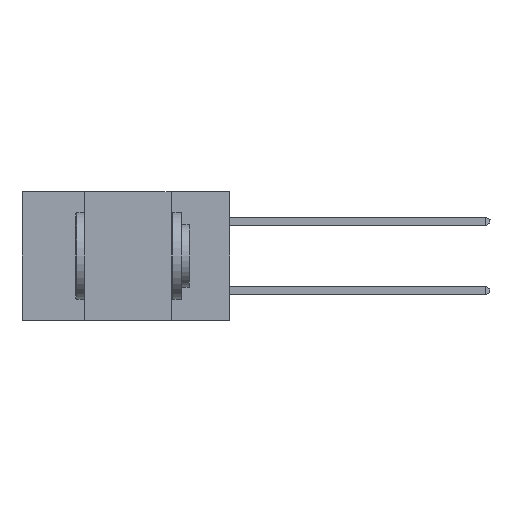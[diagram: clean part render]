
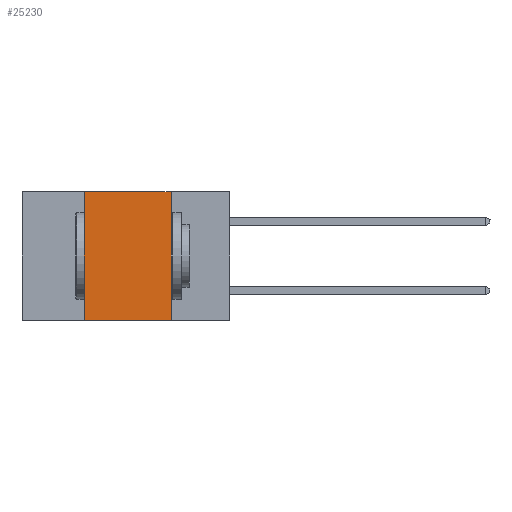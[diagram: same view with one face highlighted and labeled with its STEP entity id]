
A CAD part, left-side view. The second image highlights one B-rep face of the part: STEP entity #25230.
In plain terms, the highlighted planar face has unit normal (-1, 0, 0).
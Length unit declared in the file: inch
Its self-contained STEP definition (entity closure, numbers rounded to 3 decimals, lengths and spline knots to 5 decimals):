
#1591 = CARTESIAN_POINT ( 'NONE',  ( 0., 0.42, 0. ) ) ;
#3230 = VECTOR ( 'NONE', #23755, 39.37008 ) ;
#4613 = EDGE_LOOP ( 'NONE', ( #8569, #6033, #12265, #22360 ) ) ;
#5882 = VECTOR ( 'NONE', #16762, 39.37008 ) ;
#6033 = ORIENTED_EDGE ( 'NONE', *, *, #14256, .F. ) ;
#6796 = CARTESIAN_POINT ( 'NONE',  ( 0., 0.42, 0. ) ) ;
#7136 = VERTEX_POINT ( 'NONE', #1591 ) ;
#8569 = ORIENTED_EDGE ( 'NONE', *, *, #26281, .F. ) ;
#9524 = VECTOR ( 'NONE', #10035, 39.37008 ) ;
#10035 = DIRECTION ( 'NONE',  ( 0., -1., 0. ) ) ;
#10051 = VECTOR ( 'NONE', #17289, 39.37008 ) ;
#10116 = CARTESIAN_POINT ( 'NONE',  ( 0., 0.6, -0.37 ) ) ;
#10561 = EDGE_CURVE ( 'NONE', #14721, #21304, #23443, .T. ) ;
#10604 = FACE_OUTER_BOUND ( 'NONE', #4613, .T. ) ;
#11136 = DIRECTION ( 'NONE',  ( 0., 0., -1. ) ) ;
#11238 = DIRECTION ( 'NONE',  ( 1., 0., 0. ) ) ;
#11724 = LINE ( 'NONE', #6796, #10051 ) ;
#12265 = ORIENTED_EDGE ( 'NONE', *, *, #18954, .F. ) ;
#14220 = LINE ( 'NONE', #25382, #5882 ) ;
#14256 = EDGE_CURVE ( 'NONE', #7136, #16171, #24878, .T. ) ;
#14721 = VERTEX_POINT ( 'NONE', #25897 ) ;
#15700 = PLANE ( 'NONE',  #19353 ) ;
#16171 = VERTEX_POINT ( 'NONE', #22251 ) ;
#16762 = DIRECTION ( 'NONE',  ( 0., 0., -1. ) ) ;
#17289 = DIRECTION ( 'NONE',  ( 0., 0., 1. ) ) ;
#18954 = EDGE_CURVE ( 'NONE', #14721, #7136, #11724, .T. ) ;
#19353 = AXIS2_PLACEMENT_3D ( 'NONE', #19858, #11238, #11136 ) ;
#19409 = CARTESIAN_POINT ( 'NONE',  ( 0., 0.6, 0. ) ) ;
#19858 = CARTESIAN_POINT ( 'NONE',  ( 0., 0.6, 0. ) ) ;
#21304 = VERTEX_POINT ( 'NONE', #24115 ) ;
#22251 = CARTESIAN_POINT ( 'NONE',  ( 0., 0.17, 0. ) ) ;
#22360 = ORIENTED_EDGE ( 'NONE', *, *, #10561, .T. ) ;
#23443 = LINE ( 'NONE', #10116, #9524 ) ;
#23755 = DIRECTION ( 'NONE',  ( 0., -1., 0. ) ) ;
#24115 = CARTESIAN_POINT ( 'NONE',  ( 0., 0.17, -0.37 ) ) ;
#24878 = LINE ( 'NONE', #19409, #3230 ) ;
#25230 = ADVANCED_FACE ( 'NONE', ( #10604 ), #15700, .F. ) ;
#25382 = CARTESIAN_POINT ( 'NONE',  ( 0., 0.17, 0. ) ) ;
#25897 = CARTESIAN_POINT ( 'NONE',  ( 0., 0.42, -0.37 ) ) ;
#26281 = EDGE_CURVE ( 'NONE', #16171, #21304, #14220, .T. ) ;
